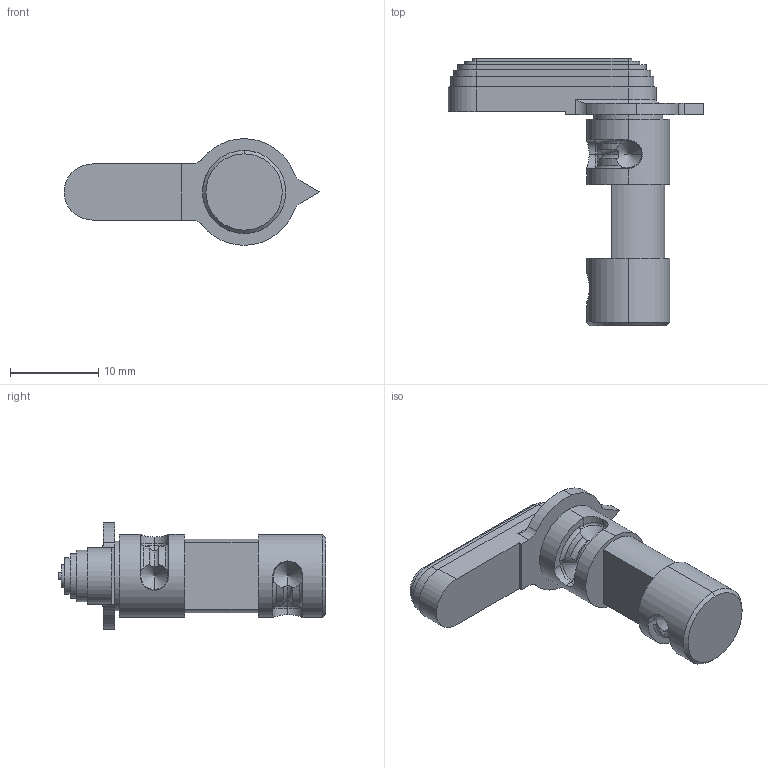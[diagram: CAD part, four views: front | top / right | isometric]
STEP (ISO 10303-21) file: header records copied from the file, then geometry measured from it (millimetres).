
FILE_DESCRIPTION (( 'STEP AP214' ), '1' );
FILE_NAME ('Fire Selector.step.step', '2019-12-18T03:07:44', ( '' ), ( '' ), 'SwSTEP 2.0', 'SolidWorks 2019', '' );
FILE_SCHEMA (( 'AUTOMOTIVE_DESIGN' ));
Length unit declared in the file: millimetre
Products named in the file (1): Fire Selector.step
Bounding box: 29.03 x 30.4 x 12.12 mm (x, y, z)
Volume: 2158.2 mm3; surface area: 1564.9 mm2
Topology: 1 solids, 1 shells, 130 faces, 316 edges, 184 vertices
Faces by surface type: plane 53, cylinder 42, torus 17, cone 10, bspline 8
Entity records: 4463 total; most frequent: CARTESIAN_POINT 1503, ORIENTED_EDGE 616, DIRECTION 613, EDGE_CURVE 308, AXIS2_PLACEMENT_3D 240, VERTEX_POINT 184, EDGE_LOOP 134, VECTOR 133
